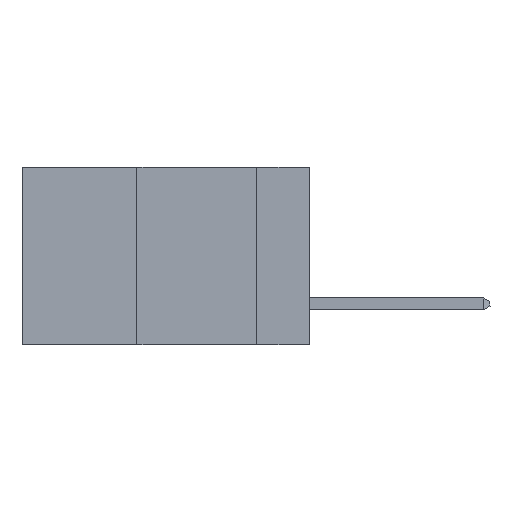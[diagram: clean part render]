
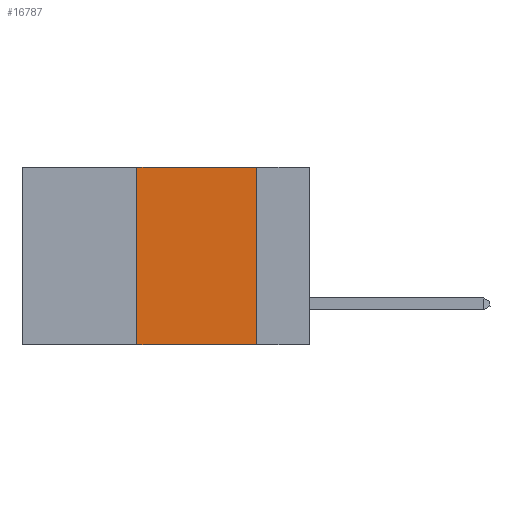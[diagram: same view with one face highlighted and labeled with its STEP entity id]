
A CAD part, left-side view. The second image highlights one B-rep face of the part: STEP entity #16787.
In plain terms, the highlighted planar face has unit normal (-1, 0, 0).
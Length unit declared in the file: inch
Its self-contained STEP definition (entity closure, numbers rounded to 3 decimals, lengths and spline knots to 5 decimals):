
#138 = CARTESIAN_POINT ( 'NONE',  ( 0., 0.6, 0. ) ) ;
#1082 = VECTOR ( 'NONE', #6857, 39.37008 ) ;
#1636 = AXIS2_PLACEMENT_3D ( 'NONE', #2634, #29120, #11579 ) ;
#2634 = CARTESIAN_POINT ( 'NONE',  ( 0., 0.6, 0. ) ) ;
#3825 = CARTESIAN_POINT ( 'NONE',  ( 0., 0.36, 0. ) ) ;
#4085 = CARTESIAN_POINT ( 'NONE',  ( 0., 0.6, -0.37 ) ) ;
#4855 = VERTEX_POINT ( 'NONE', #15089 ) ;
#6857 = DIRECTION ( 'NONE',  ( 0., 0., 1. ) ) ;
#8008 = FACE_OUTER_BOUND ( 'NONE', #17140, .T. ) ;
#8519 = PLANE ( 'NONE',  #1636 ) ;
#8701 = VECTOR ( 'NONE', #25509, 39.37008 ) ;
#9235 = CARTESIAN_POINT ( 'NONE',  ( 0., 0.36, 0. ) ) ;
#9620 = LINE ( 'NONE', #25384, #8701 ) ;
#9905 = CARTESIAN_POINT ( 'NONE',  ( 0., 0.11, -0.37 ) ) ;
#11579 = DIRECTION ( 'NONE',  ( 0., 0., -1. ) ) ;
#13805 = EDGE_CURVE ( 'NONE', #4855, #15230, #24735, .T. ) ;
#14366 = VECTOR ( 'NONE', #29564, 39.37008 ) ;
#15089 = CARTESIAN_POINT ( 'NONE',  ( 0., 0.36, -0.37 ) ) ;
#15230 = VERTEX_POINT ( 'NONE', #9905 ) ;
#15304 = LINE ( 'NONE', #138, #14366 ) ;
#15387 = ORIENTED_EDGE ( 'NONE', *, *, #30771, .F. ) ;
#16043 = VECTOR ( 'NONE', #27574, 39.37008 ) ;
#16787 = ADVANCED_FACE ( 'NONE', ( #8008 ), #8519, .F. ) ;
#17140 = EDGE_LOOP ( 'NONE', ( #20029, #26604, #15387, #30145 ) ) ;
#20029 = ORIENTED_EDGE ( 'NONE', *, *, #34876, .F. ) ;
#20309 = VERTEX_POINT ( 'NONE', #9235 ) ;
#22270 = VERTEX_POINT ( 'NONE', #25588 ) ;
#23944 = EDGE_CURVE ( 'NONE', #20309, #22270, #15304, .T. ) ;
#24550 = LINE ( 'NONE', #3825, #1082 ) ;
#24735 = LINE ( 'NONE', #4085, #16043 ) ;
#25384 = CARTESIAN_POINT ( 'NONE',  ( 0., 0.11, 0. ) ) ;
#25509 = DIRECTION ( 'NONE',  ( 0., 0., -1. ) ) ;
#25588 = CARTESIAN_POINT ( 'NONE',  ( 0., 0.11, 0. ) ) ;
#26604 = ORIENTED_EDGE ( 'NONE', *, *, #23944, .F. ) ;
#27574 = DIRECTION ( 'NONE',  ( 0., -1., 0. ) ) ;
#29120 = DIRECTION ( 'NONE',  ( 1., 0., 0. ) ) ;
#29564 = DIRECTION ( 'NONE',  ( 0., -1., 0. ) ) ;
#30145 = ORIENTED_EDGE ( 'NONE', *, *, #13805, .T. ) ;
#30771 = EDGE_CURVE ( 'NONE', #4855, #20309, #24550, .T. ) ;
#34876 = EDGE_CURVE ( 'NONE', #22270, #15230, #9620, .T. ) ;
